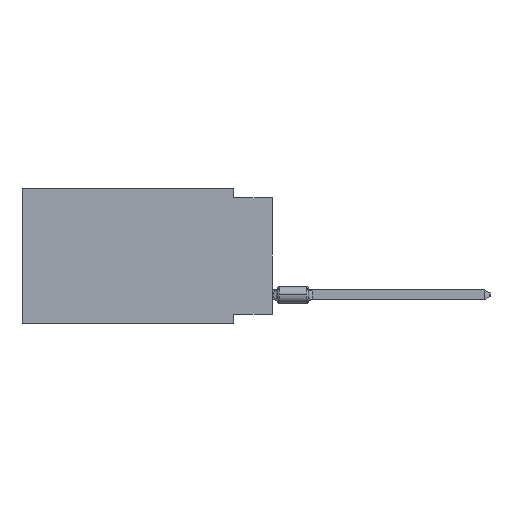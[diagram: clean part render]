
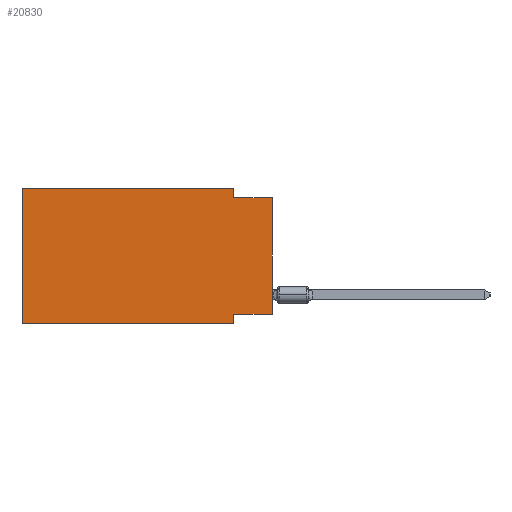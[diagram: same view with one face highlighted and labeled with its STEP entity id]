
A CAD part, left-side view. The second image highlights one B-rep face of the part: STEP entity #20830.
In plain terms, the highlighted planar face has unit normal (-1, 0, 0).
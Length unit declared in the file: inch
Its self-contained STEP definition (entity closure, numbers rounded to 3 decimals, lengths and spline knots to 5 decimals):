
#928 = EDGE_CURVE ( 'NONE', #44251, #90736, #93156, .T. ) ;
#3829 = CARTESIAN_POINT ( 'NONE',  ( 0., 0., -0.325 ) ) ;
#4007 = DIRECTION ( 'NONE',  ( 1., 0., 0. ) ) ;
#4833 = LINE ( 'NONE', #74715, #99443 ) ;
#4933 = LINE ( 'NONE', #39321, #104389 ) ;
#5508 = DIRECTION ( 'NONE',  ( 0., -1., 0. ) ) ;
#6106 = LINE ( 'NONE', #102892, #15456 ) ;
#8923 = DIRECTION ( 'NONE',  ( 0., 0., -1. ) ) ;
#9985 = VECTOR ( 'NONE', #70538, 39.37008 ) ;
#12338 = VECTOR ( 'NONE', #87065, 39.37008 ) ;
#12976 = CARTESIAN_POINT ( 'NONE',  ( 0., 0.1, -0.35 ) ) ;
#15357 = VECTOR ( 'NONE', #8923, 39.37008 ) ;
#15456 = VECTOR ( 'NONE', #49660, 39.37008 ) ;
#19796 = ORIENTED_EDGE ( 'NONE', *, *, #37717, .T. ) ;
#20830 = ADVANCED_FACE ( 'NONE', ( #83101 ), #65903, .F. ) ;
#22319 = CARTESIAN_POINT ( 'NONE',  ( 0., 0.645, 0. ) ) ;
#23796 = CARTESIAN_POINT ( 'NONE',  ( 0., 0., -0.025 ) ) ;
#24016 = CARTESIAN_POINT ( 'NONE',  ( 0., 0.1, -0.025 ) ) ;
#25275 = LINE ( 'NONE', #95163, #9985 ) ;
#29603 = VECTOR ( 'NONE', #5508, 39.37008 ) ;
#36328 = VERTEX_POINT ( 'NONE', #105907 ) ;
#37717 = EDGE_CURVE ( 'NONE', #93577, #90736, #78056, .T. ) ;
#39321 = CARTESIAN_POINT ( 'NONE',  ( 0., 0.645, 0. ) ) ;
#39870 = DIRECTION ( 'NONE',  ( 0., 0., 1. ) ) ;
#41154 = CARTESIAN_POINT ( 'NONE',  ( 0., 0.1, 0. ) ) ;
#43520 = LINE ( 'NONE', #45216, #12338 ) ;
#43652 = DIRECTION ( 'NONE',  ( 0., 0., 1. ) ) ;
#44251 = VERTEX_POINT ( 'NONE', #24016 ) ;
#45216 = CARTESIAN_POINT ( 'NONE',  ( 0., 0., -0.325 ) ) ;
#45627 = VERTEX_POINT ( 'NONE', #54279 ) ;
#49660 = DIRECTION ( 'NONE',  ( 0., -1., 0. ) ) ;
#51285 = ORIENTED_EDGE ( 'NONE', *, *, #928, .F. ) ;
#52478 = LINE ( 'NONE', #87392, #15357 ) ;
#54279 = CARTESIAN_POINT ( 'NONE',  ( 0., 0.645, -0.35 ) ) ;
#56953 = DIRECTION ( 'NONE',  ( 0., -1., 0. ) ) ;
#61656 = EDGE_CURVE ( 'NONE', #45627, #71237, #4933, .T. ) ;
#64952 = AXIS2_PLACEMENT_3D ( 'NONE', #22319, #4007, #91124 ) ;
#65903 = PLANE ( 'NONE',  #64952 ) ;
#66053 = VERTEX_POINT ( 'NONE', #41154 ) ;
#69458 = CARTESIAN_POINT ( 'NONE',  ( 0., 0., 0. ) ) ;
#70538 = DIRECTION ( 'NONE',  ( 0., 0., -1. ) ) ;
#71237 = VERTEX_POINT ( 'NONE', #111967 ) ;
#74123 = ORIENTED_EDGE ( 'NONE', *, *, #79702, .F. ) ;
#74715 = CARTESIAN_POINT ( 'NONE',  ( 0., 0.645, 0. ) ) ;
#78056 = LINE ( 'NONE', #69458, #83759 ) ;
#78910 = EDGE_LOOP ( 'NONE', ( #19796, #51285, #100346, #106785, #92788, #82499, #80591, #74123 ) ) ;
#79702 = EDGE_CURVE ( 'NONE', #93577, #36328, #43520, .T. ) ;
#80591 = ORIENTED_EDGE ( 'NONE', *, *, #105014, .F. ) ;
#82499 = ORIENTED_EDGE ( 'NONE', *, *, #98800, .T. ) ;
#83101 = FACE_OUTER_BOUND ( 'NONE', #78910, .T. ) ;
#83759 = VECTOR ( 'NONE', #43652, 39.37008 ) ;
#87065 = DIRECTION ( 'NONE',  ( 0., 1., 0. ) ) ;
#87392 = CARTESIAN_POINT ( 'NONE',  ( 0., 0.1, 0. ) ) ;
#90736 = VERTEX_POINT ( 'NONE', #91785 ) ;
#91124 = DIRECTION ( 'NONE',  ( 0., 0., -1. ) ) ;
#91785 = CARTESIAN_POINT ( 'NONE',  ( 0., 0., -0.025 ) ) ;
#92788 = ORIENTED_EDGE ( 'NONE', *, *, #61656, .F. ) ;
#93156 = LINE ( 'NONE', #23796, #29603 ) ;
#93577 = VERTEX_POINT ( 'NONE', #3829 ) ;
#95163 = CARTESIAN_POINT ( 'NONE',  ( 0., 0.1, -0.35 ) ) ;
#97929 = EDGE_CURVE ( 'NONE', #66053, #44251, #52478, .T. ) ;
#98800 = EDGE_CURVE ( 'NONE', #45627, #102102, #6106, .T. ) ;
#99443 = VECTOR ( 'NONE', #56953, 39.37008 ) ;
#100346 = ORIENTED_EDGE ( 'NONE', *, *, #97929, .F. ) ;
#102102 = VERTEX_POINT ( 'NONE', #12976 ) ;
#102488 = EDGE_CURVE ( 'NONE', #71237, #66053, #4833, .T. ) ;
#102892 = CARTESIAN_POINT ( 'NONE',  ( 0., 0.645, -0.35 ) ) ;
#104389 = VECTOR ( 'NONE', #39870, 39.37008 ) ;
#105014 = EDGE_CURVE ( 'NONE', #36328, #102102, #25275, .T. ) ;
#105907 = CARTESIAN_POINT ( 'NONE',  ( 0., 0.1, -0.325 ) ) ;
#106785 = ORIENTED_EDGE ( 'NONE', *, *, #102488, .F. ) ;
#111967 = CARTESIAN_POINT ( 'NONE',  ( 0., 0.645, 0. ) ) ;
